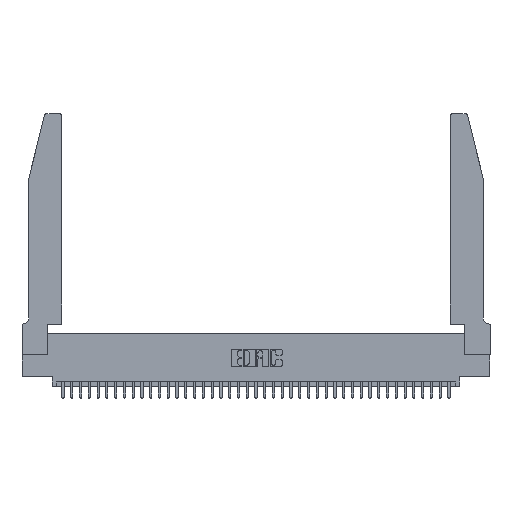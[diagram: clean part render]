
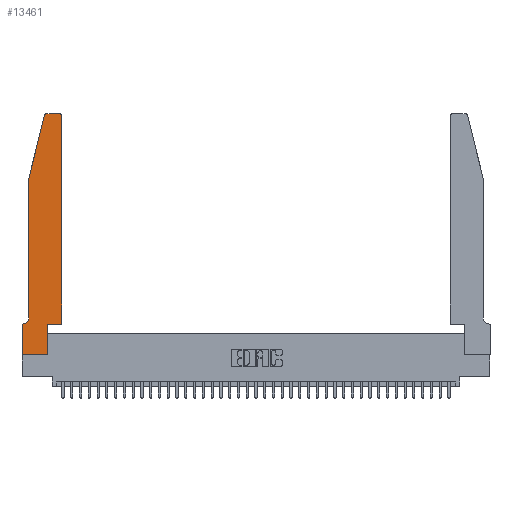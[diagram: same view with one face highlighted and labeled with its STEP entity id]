
A CAD part, top view. The second image highlights one B-rep face of the part: STEP entity #13461.
In plain terms, the highlighted planar face has unit normal (0, 0, 1).
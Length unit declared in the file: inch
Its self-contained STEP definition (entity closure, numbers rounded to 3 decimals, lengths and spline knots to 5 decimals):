
#76 = CARTESIAN_POINT ( 'NONE',  ( 0.4505, 0.35, 0.37 ) ) ;
#285 = ORIENTED_EDGE ( 'NONE', *, *, #5296, .T. ) ;
#813 = ORIENTED_EDGE ( 'NONE', *, *, #35669, .T. ) ;
#888 = VECTOR ( 'NONE', #34737, 39.37008 ) ;
#993 = VERTEX_POINT ( 'NONE', #31920 ) ;
#2346 = VECTOR ( 'NONE', #13975, 39.37008 ) ;
#2696 = DIRECTION ( 'NONE',  ( 1., 0., 0. ) ) ;
#3254 = CARTESIAN_POINT ( 'NONE',  ( 0.25487, 2.72718, 0.37 ) ) ;
#4480 = DIRECTION ( 'NONE',  ( 1., 0., 0. ) ) ;
#5178 = EDGE_CURVE ( 'NONE', #31635, #30631, #21565, .T. ) ;
#5296 = EDGE_CURVE ( 'NONE', #993, #32085, #17195, .T. ) ;
#6507 = CARTESIAN_POINT ( 'NONE',  ( 0.0755, 0.42, 0.37 ) ) ;
#6604 = LINE ( 'NONE', #39154, #30188 ) ;
#6891 = VERTEX_POINT ( 'NONE', #11213 ) ;
#7131 = VECTOR ( 'NONE', #4480, 39.37008 ) ;
#7325 = ORIENTED_EDGE ( 'NONE', *, *, #38000, .T. ) ;
#7702 = ORIENTED_EDGE ( 'NONE', *, *, #29983, .T. ) ;
#8298 = ORIENTED_EDGE ( 'NONE', *, *, #19708, .T. ) ;
#9304 = VERTEX_POINT ( 'NONE', #24368 ) ;
#9703 = EDGE_CURVE ( 'NONE', #31910, #9304, #17892, .T. ) ;
#10047 = DIRECTION ( 'NONE',  ( 0., 0., 1. ) ) ;
#10730 = EDGE_CURVE ( 'NONE', #6891, #18435, #39563, .T. ) ;
#10866 = CARTESIAN_POINT ( 'NONE',  ( 0.4205, 2.75, 0.37 ) ) ;
#10971 = ORIENTED_EDGE ( 'NONE', *, *, #5178, .T. ) ;
#11213 = CARTESIAN_POINT ( 'NONE',  ( 0.2865, 0., 0.37 ) ) ;
#11715 = CIRCLE ( 'NONE', #33528, 0.03 ) ;
#11791 = DIRECTION ( 'NONE',  ( 0., 0., 1. ) ) ;
#11928 = CARTESIAN_POINT ( 'NONE',  ( 0., 0.35, 0.37 ) ) ;
#13127 = DIRECTION ( 'NONE',  ( 1., 0., 0. ) ) ;
#13141 = DIRECTION ( 'NONE',  ( -1., 0., 0. ) ) ;
#13461 = ADVANCED_FACE ( 'NONE', ( #19154 ), #14360, .T. ) ;
#13673 = CARTESIAN_POINT ( 'NONE',  ( 0.0755, 0.35, 0.37 ) ) ;
#13975 = DIRECTION ( 'NONE',  ( 0., -1., 0. ) ) ;
#13993 = CIRCLE ( 'NONE', #30617, 0.07 ) ;
#14185 = EDGE_CURVE ( 'NONE', #18435, #31910, #21540, .T. ) ;
#14360 = PLANE ( 'NONE',  #26094 ) ;
#15768 = VECTOR ( 'NONE', #22947, 39.37008 ) ;
#15858 = DIRECTION ( 'NONE',  ( -1., 0., 0. ) ) ;
#16130 = DIRECTION ( 'NONE',  ( 0., 1., 0. ) ) ;
#16723 = ORIENTED_EDGE ( 'NONE', *, *, #14185, .T. ) ;
#16785 = CARTESIAN_POINT ( 'NONE',  ( 0.4505, 0.35, 0.37 ) ) ;
#17195 = LINE ( 'NONE', #22220, #888 ) ;
#17391 = EDGE_CURVE ( 'NONE', #9304, #26145, #11715, .T. ) ;
#17838 = LINE ( 'NONE', #18378, #24145 ) ;
#17892 = LINE ( 'NONE', #36071, #37686 ) ;
#18378 = CARTESIAN_POINT ( 'NONE',  ( 0.0755, 2., 0.37 ) ) ;
#18435 = VERTEX_POINT ( 'NONE', #36062 ) ;
#18480 = EDGE_CURVE ( 'NONE', #25854, #993, #17838, .T. ) ;
#19154 = FACE_OUTER_BOUND ( 'NONE', #39535, .T. ) ;
#19190 = DIRECTION ( 'NONE',  ( 0., 0., -1. ) ) ;
#19708 = EDGE_CURVE ( 'NONE', #30631, #6891, #6604, .T. ) ;
#19825 = CARTESIAN_POINT ( 'NONE',  ( 0.2605, 2.75, 0.37 ) ) ;
#20517 = CARTESIAN_POINT ( 'NONE',  ( 0., 0., 0.37 ) ) ;
#20702 = CARTESIAN_POINT ( 'NONE',  ( 0.284, 2.72, 0.37 ) ) ;
#21224 = VECTOR ( 'NONE', #25796, 39.37008 ) ;
#21540 = LINE ( 'NONE', #16785, #7131 ) ;
#21565 = LINE ( 'NONE', #32284, #2346 ) ;
#22220 = CARTESIAN_POINT ( 'NONE',  ( 0.0755, 2., 0.37 ) ) ;
#22565 = CARTESIAN_POINT ( 'NONE',  ( 0.2865, 0.35, 0.37 ) ) ;
#22744 = ORIENTED_EDGE ( 'NONE', *, *, #9703, .T. ) ;
#22947 = DIRECTION ( 'NONE',  ( -1., 0., 0. ) ) ;
#23651 = CIRCLE ( 'NONE', #27885, 0.03 ) ;
#24145 = VECTOR ( 'NONE', #34028, 39.37008 ) ;
#24368 = CARTESIAN_POINT ( 'NONE',  ( 0.4505, 2.72, 0.37 ) ) ;
#25175 = LINE ( 'NONE', #13673, #36716 ) ;
#25542 = CARTESIAN_POINT ( 'NONE',  ( 0.0055, 0.42, 0.37 ) ) ;
#25796 = DIRECTION ( 'NONE',  ( 0., 1., 0. ) ) ;
#25854 = VERTEX_POINT ( 'NONE', #3254 ) ;
#26094 = AXIS2_PLACEMENT_3D ( 'NONE', #11928, #11791, #2696 ) ;
#26145 = VERTEX_POINT ( 'NONE', #10866 ) ;
#26148 = EDGE_CURVE ( 'NONE', #26145, #26424, #36961, .T. ) ;
#26424 = VERTEX_POINT ( 'NONE', #33297 ) ;
#26881 = ORIENTED_EDGE ( 'NONE', *, *, #10730, .T. ) ;
#27361 = VERTEX_POINT ( 'NONE', #27983 ) ;
#27885 = AXIS2_PLACEMENT_3D ( 'NONE', #20702, #29877, #29610 ) ;
#27983 = CARTESIAN_POINT ( 'NONE',  ( 0.0055, 0.35, 0.37 ) ) ;
#28467 = CARTESIAN_POINT ( 'NONE',  ( 0.4205, 2.72, 0.37 ) ) ;
#28819 = ORIENTED_EDGE ( 'NONE', *, *, #26148, .T. ) ;
#29610 = DIRECTION ( 'NONE',  ( 1., 0., 0. ) ) ;
#29877 = DIRECTION ( 'NONE',  ( 0., 0., 1. ) ) ;
#29983 = EDGE_CURVE ( 'NONE', #26424, #25854, #23651, .T. ) ;
#30188 = VECTOR ( 'NONE', #32938, 39.37008 ) ;
#30617 = AXIS2_PLACEMENT_3D ( 'NONE', #25542, #19190, #15858 ) ;
#30631 = VERTEX_POINT ( 'NONE', #20517 ) ;
#31635 = VERTEX_POINT ( 'NONE', #34283 ) ;
#31910 = VERTEX_POINT ( 'NONE', #76 ) ;
#31920 = CARTESIAN_POINT ( 'NONE',  ( 0.0755, 2., 0.37 ) ) ;
#32085 = VERTEX_POINT ( 'NONE', #6507 ) ;
#32284 = CARTESIAN_POINT ( 'NONE',  ( 0., 0., 0.37 ) ) ;
#32938 = DIRECTION ( 'NONE',  ( 1., 0., 0. ) ) ;
#33297 = CARTESIAN_POINT ( 'NONE',  ( 0.284, 2.75, 0.37 ) ) ;
#33528 = AXIS2_PLACEMENT_3D ( 'NONE', #28467, #10047, #13127 ) ;
#34028 = DIRECTION ( 'NONE',  ( -0.239, -0.971, 0. ) ) ;
#34283 = CARTESIAN_POINT ( 'NONE',  ( 0., 0.35, 0.37 ) ) ;
#34737 = DIRECTION ( 'NONE',  ( 0., -1., 0. ) ) ;
#35669 = EDGE_CURVE ( 'NONE', #27361, #31635, #25175, .T. ) ;
#36062 = CARTESIAN_POINT ( 'NONE',  ( 0.2865, 0.35, 0.37 ) ) ;
#36071 = CARTESIAN_POINT ( 'NONE',  ( 0.4505, 0.35, 0.37 ) ) ;
#36650 = ORIENTED_EDGE ( 'NONE', *, *, #18480, .T. ) ;
#36716 = VECTOR ( 'NONE', #13141, 39.37008 ) ;
#36961 = LINE ( 'NONE', #19825, #15768 ) ;
#37686 = VECTOR ( 'NONE', #16130, 39.37008 ) ;
#38000 = EDGE_CURVE ( 'NONE', #32085, #27361, #13993, .T. ) ;
#39071 = ORIENTED_EDGE ( 'NONE', *, *, #17391, .T. ) ;
#39154 = CARTESIAN_POINT ( 'NONE',  ( 0., 0., 0.37 ) ) ;
#39535 = EDGE_LOOP ( 'NONE', ( #28819, #7702, #36650, #285, #7325, #813, #10971, #8298, #26881, #16723, #22744, #39071 ) ) ;
#39563 = LINE ( 'NONE', #22565, #21224 ) ;
